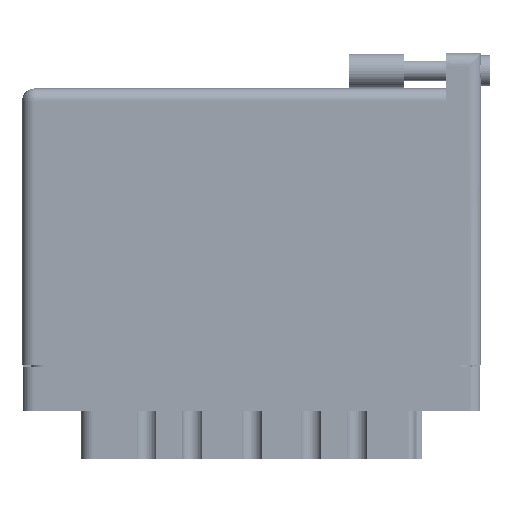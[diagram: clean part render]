
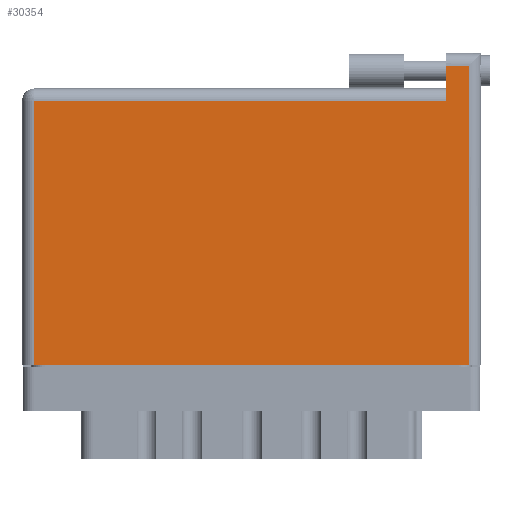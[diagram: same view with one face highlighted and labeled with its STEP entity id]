
A CAD part, front view. The second image highlights one B-rep face of the part: STEP entity #30354.
In plain terms, the highlighted face is planar.
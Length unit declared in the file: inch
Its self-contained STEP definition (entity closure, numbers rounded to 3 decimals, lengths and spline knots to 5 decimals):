
#1273 = EDGE_CURVE ( 'NONE', #4205, #20083, #31113, .T. ) ;
#2438 = CARTESIAN_POINT ( 'NONE',  ( 2.403, 1.496, 0. ) ) ;
#4205 = VERTEX_POINT ( 'NONE', #49360 ) ;
#5126 = CARTESIAN_POINT ( 'NONE',  ( 2.53, 0., 0. ) ) ;
#6222 = EDGE_LOOP ( 'NONE', ( #45535, #10508, #27184, #39320, #30666, #18080 ) ) ;
#9062 = LINE ( 'NONE', #43964, #37402 ) ;
#10013 = LINE ( 'NONE', #36532, #21655 ) ;
#10508 = ORIENTED_EDGE ( 'NONE', *, *, #37683, .T. ) ;
#11161 = LINE ( 'NONE', #50711, #43416 ) ;
#14478 = DIRECTION ( 'NONE',  ( -1., 0., 0. ) ) ;
#16153 = EDGE_CURVE ( 'NONE', #49380, #24806, #10013, .T. ) ;
#16188 = DIRECTION ( 'NONE',  ( 0., -1., 0. ) ) ;
#18080 = ORIENTED_EDGE ( 'NONE', *, *, #1273, .T. ) ;
#19073 = VECTOR ( 'NONE', #28501, 39.37008 ) ;
#20083 = VERTEX_POINT ( 'NONE', #20616 ) ;
#20388 = CARTESIAN_POINT ( 'NONE',  ( 2.53, 1.696, 0. ) ) ;
#20616 = CARTESIAN_POINT ( 'NONE',  ( 0.07, 0., 0. ) ) ;
#20738 = EDGE_CURVE ( 'NONE', #20083, #21527, #31966, .T. ) ;
#21527 = VERTEX_POINT ( 'NONE', #5126 ) ;
#21655 = VECTOR ( 'NONE', #16188, 39.37008 ) ;
#22258 = VECTOR ( 'NONE', #14478, 39.37008 ) ;
#24030 = CARTESIAN_POINT ( 'NONE',  ( 0., 1.566, 0. ) ) ;
#24806 = VERTEX_POINT ( 'NONE', #2438 ) ;
#25842 = VERTEX_POINT ( 'NONE', #20388 ) ;
#26714 = FACE_OUTER_BOUND ( 'NONE', #6222, .T. ) ;
#27184 = ORIENTED_EDGE ( 'NONE', *, *, #30681, .T. ) ;
#28501 = DIRECTION ( 'NONE',  ( 1., 0., 0. ) ) ;
#29131 = CARTESIAN_POINT ( 'NONE',  ( 0.07, 0., 0. ) ) ;
#30354 = ADVANCED_FACE ( 'NONE', ( #26714 ), #45291, .F. ) ;
#30666 = ORIENTED_EDGE ( 'NONE', *, *, #45320, .T. ) ;
#30681 = EDGE_CURVE ( 'NONE', #25842, #49380, #11161, .T. ) ;
#31113 = LINE ( 'NONE', #29131, #50512 ) ;
#31300 = LINE ( 'NONE', #43527, #22258 ) ;
#31966 = LINE ( 'NONE', #33139, #19073 ) ;
#32645 = DIRECTION ( 'NONE',  ( -1., 0., 0. ) ) ;
#32904 = DIRECTION ( 'NONE',  ( 0., -1., 0. ) ) ;
#33139 = CARTESIAN_POINT ( 'NONE',  ( 0., 0., 0. ) ) ;
#34212 = DIRECTION ( 'NONE',  ( -1., 0., 0. ) ) ;
#36532 = CARTESIAN_POINT ( 'NONE',  ( 2.403, 1.766, 0. ) ) ;
#37402 = VECTOR ( 'NONE', #40312, 39.37008 ) ;
#37683 = EDGE_CURVE ( 'NONE', #21527, #25842, #9062, .T. ) ;
#39320 = ORIENTED_EDGE ( 'NONE', *, *, #16153, .T. ) ;
#40312 = DIRECTION ( 'NONE',  ( 0., 1., 0. ) ) ;
#42880 = AXIS2_PLACEMENT_3D ( 'NONE', #24030, #52909, #32645 ) ;
#43416 = VECTOR ( 'NONE', #34212, 39.37008 ) ;
#43527 = CARTESIAN_POINT ( 'NONE',  ( 0., 1.496, 0. ) ) ;
#43964 = CARTESIAN_POINT ( 'NONE',  ( 2.53, 1.766, 0. ) ) ;
#45291 = PLANE ( 'NONE',  #42880 ) ;
#45320 = EDGE_CURVE ( 'NONE', #24806, #4205, #31300, .T. ) ;
#45535 = ORIENTED_EDGE ( 'NONE', *, *, #20738, .T. ) ;
#47879 = CARTESIAN_POINT ( 'NONE',  ( 2.403, 1.696, 0. ) ) ;
#49360 = CARTESIAN_POINT ( 'NONE',  ( 0.07, 1.496, 0. ) ) ;
#49380 = VERTEX_POINT ( 'NONE', #47879 ) ;
#50512 = VECTOR ( 'NONE', #32904, 39.37008 ) ;
#50711 = CARTESIAN_POINT ( 'NONE',  ( 0., 1.696, 0. ) ) ;
#52909 = DIRECTION ( 'NONE',  ( 0., 0., -1. ) ) ;
